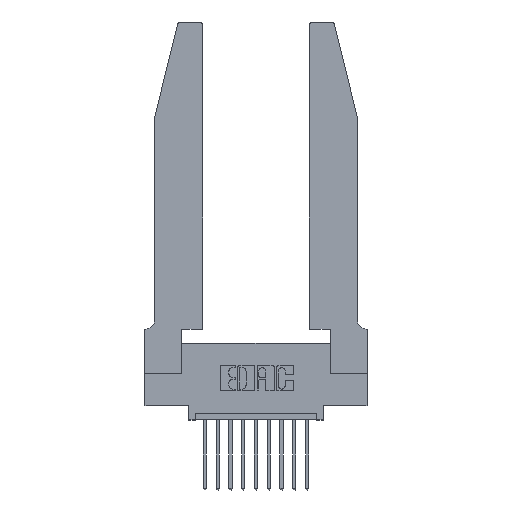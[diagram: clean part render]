
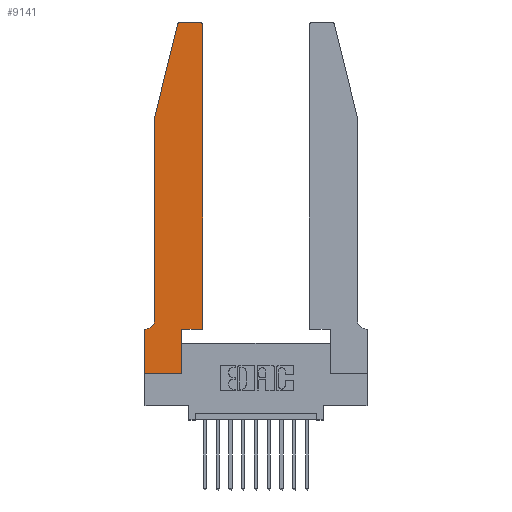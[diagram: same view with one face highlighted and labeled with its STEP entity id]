
A CAD part, top view. The second image highlights one B-rep face of the part: STEP entity #9141.
In plain terms, the highlighted planar face has unit normal (0, 0, 1).
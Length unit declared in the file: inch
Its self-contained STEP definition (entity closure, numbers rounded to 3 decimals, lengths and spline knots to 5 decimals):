
#123 = VECTOR ( 'NONE', #8610, 39.37008 ) ;
#129 = DIRECTION ( 'NONE',  ( -0.239, -0.971, 0. ) ) ;
#259 = ORIENTED_EDGE ( 'NONE', *, *, #3892, .T. ) ;
#424 = AXIS2_PLACEMENT_3D ( 'NONE', #13487, #7077, #10950 ) ;
#572 = EDGE_CURVE ( 'NONE', #2619, #15729, #4001, .T. ) ;
#602 = LINE ( 'NONE', #15996, #10327 ) ;
#708 = CARTESIAN_POINT ( 'NONE',  ( 0.0755, 0.42, 0.37 ) ) ;
#1080 = EDGE_CURVE ( 'NONE', #6767, #2516, #15290, .T. ) ;
#1112 = DIRECTION ( 'NONE',  ( 0., -1., 0. ) ) ;
#1384 = ORIENTED_EDGE ( 'NONE', *, *, #2232, .T. ) ;
#1392 = CARTESIAN_POINT ( 'NONE',  ( 0.284, 2.75, 0.37 ) ) ;
#1560 = CARTESIAN_POINT ( 'NONE',  ( 0.0055, 0.35, 0.37 ) ) ;
#1568 = VERTEX_POINT ( 'NONE', #708 ) ;
#1604 = VECTOR ( 'NONE', #12447, 39.37008 ) ;
#2035 = CARTESIAN_POINT ( 'NONE',  ( 0.0755, 2., 0.37 ) ) ;
#2090 = EDGE_CURVE ( 'NONE', #6805, #8335, #14498, .T. ) ;
#2190 = CARTESIAN_POINT ( 'NONE',  ( 0.4505, 0.35, 0.37 ) ) ;
#2211 = EDGE_LOOP ( 'NONE', ( #6377, #2398, #7430, #259, #9019, #11059, #11183, #1384, #7874, #5995, #8730, #14293 ) ) ;
#2232 = EDGE_CURVE ( 'NONE', #2516, #8833, #6122, .T. ) ;
#2398 = ORIENTED_EDGE ( 'NONE', *, *, #12355, .T. ) ;
#2414 = VECTOR ( 'NONE', #3822, 39.37008 ) ;
#2433 = LINE ( 'NONE', #3524, #16094 ) ;
#2443 = CARTESIAN_POINT ( 'NONE',  ( 0.25487, 2.72718, 0.37 ) ) ;
#2489 = CARTESIAN_POINT ( 'NONE',  ( 0.0755, 0.35, 0.37 ) ) ;
#2516 = VERTEX_POINT ( 'NONE', #11698 ) ;
#2619 = VERTEX_POINT ( 'NONE', #15563 ) ;
#2877 = DIRECTION ( 'NONE',  ( 0., 0., 1. ) ) ;
#2890 = EDGE_CURVE ( 'NONE', #13653, #11771, #15838, .T. ) ;
#3061 = CARTESIAN_POINT ( 'NONE',  ( 0.0055, 0.42, 0.37 ) ) ;
#3179 = DIRECTION ( 'NONE',  ( 0., -1., 0. ) ) ;
#3524 = CARTESIAN_POINT ( 'NONE',  ( 0.2865, 0.35, 0.37 ) ) ;
#3822 = DIRECTION ( 'NONE',  ( -1., 0., 0. ) ) ;
#3892 = EDGE_CURVE ( 'NONE', #11771, #1568, #602, .T. ) ;
#4001 = LINE ( 'NONE', #2190, #4210 ) ;
#4210 = VECTOR ( 'NONE', #12067, 39.37008 ) ;
#4375 = VECTOR ( 'NONE', #3179, 39.37008 ) ;
#4435 = DIRECTION ( 'NONE',  ( 0., 0., -1. ) ) ;
#4897 = AXIS2_PLACEMENT_3D ( 'NONE', #3061, #4435, #8191 ) ;
#5156 = VECTOR ( 'NONE', #15316, 39.37008 ) ;
#5210 = AXIS2_PLACEMENT_3D ( 'NONE', #15967, #7349, #8511 ) ;
#5339 = PLANE ( 'NONE',  #11148 ) ;
#5579 = CARTESIAN_POINT ( 'NONE',  ( 0.4205, 2.75, 0.37 ) ) ;
#5995 = ORIENTED_EDGE ( 'NONE', *, *, #572, .T. ) ;
#6122 = LINE ( 'NONE', #15006, #1604 ) ;
#6377 = ORIENTED_EDGE ( 'NONE', *, *, #6647, .T. ) ;
#6529 = LINE ( 'NONE', #6587, #5156 ) ;
#6587 = CARTESIAN_POINT ( 'NONE',  ( 0.4505, 0.35, 0.37 ) ) ;
#6647 = EDGE_CURVE ( 'NONE', #8335, #8070, #15917, .T. ) ;
#6732 = EDGE_CURVE ( 'NONE', #8833, #2619, #2433, .T. ) ;
#6767 = VERTEX_POINT ( 'NONE', #12322 ) ;
#6805 = VERTEX_POINT ( 'NONE', #12632 ) ;
#7077 = DIRECTION ( 'NONE',  ( 0., 0., 1. ) ) ;
#7330 = CARTESIAN_POINT ( 'NONE',  ( 0.2605, 2.75, 0.37 ) ) ;
#7349 = DIRECTION ( 'NONE',  ( 0., 0., 1. ) ) ;
#7430 = ORIENTED_EDGE ( 'NONE', *, *, #2890, .T. ) ;
#7783 = CARTESIAN_POINT ( 'NONE',  ( 0., 0.35, 0.37 ) ) ;
#7874 = ORIENTED_EDGE ( 'NONE', *, *, #6732, .T. ) ;
#7917 = CIRCLE ( 'NONE', #4897, 0.07 ) ;
#8070 = VERTEX_POINT ( 'NONE', #1392 ) ;
#8191 = DIRECTION ( 'NONE',  ( -1., 0., 0. ) ) ;
#8335 = VERTEX_POINT ( 'NONE', #5579 ) ;
#8511 = DIRECTION ( 'NONE',  ( 1., 0., 0. ) ) ;
#8610 = DIRECTION ( 'NONE',  ( -1., 0., 0. ) ) ;
#8642 = VERTEX_POINT ( 'NONE', #1560 ) ;
#8700 = CARTESIAN_POINT ( 'NONE',  ( 0.0755, 2., 0.37 ) ) ;
#8730 = ORIENTED_EDGE ( 'NONE', *, *, #10810, .T. ) ;
#8820 = CIRCLE ( 'NONE', #5210, 0.03 ) ;
#8833 = VERTEX_POINT ( 'NONE', #15990 ) ;
#9019 = ORIENTED_EDGE ( 'NONE', *, *, #9876, .T. ) ;
#9141 = ADVANCED_FACE ( 'NONE', ( #10471 ), #5339, .T. ) ;
#9393 = CARTESIAN_POINT ( 'NONE',  ( 0., 0., 0.37 ) ) ;
#9876 = EDGE_CURVE ( 'NONE', #1568, #8642, #7917, .T. ) ;
#9982 = VECTOR ( 'NONE', #129, 39.37008 ) ;
#10327 = VECTOR ( 'NONE', #1112, 39.37008 ) ;
#10471 = FACE_OUTER_BOUND ( 'NONE', #2211, .T. ) ;
#10810 = EDGE_CURVE ( 'NONE', #15729, #6805, #6529, .T. ) ;
#10950 = DIRECTION ( 'NONE',  ( 1., 0., 0. ) ) ;
#11059 = ORIENTED_EDGE ( 'NONE', *, *, #16037, .T. ) ;
#11148 = AXIS2_PLACEMENT_3D ( 'NONE', #7783, #2877, #12844 ) ;
#11183 = ORIENTED_EDGE ( 'NONE', *, *, #1080, .T. ) ;
#11454 = CARTESIAN_POINT ( 'NONE',  ( 0.4505, 0.35, 0.37 ) ) ;
#11698 = CARTESIAN_POINT ( 'NONE',  ( 0., 0., 0.37 ) ) ;
#11771 = VERTEX_POINT ( 'NONE', #2035 ) ;
#12067 = DIRECTION ( 'NONE',  ( 1., 0., 0. ) ) ;
#12322 = CARTESIAN_POINT ( 'NONE',  ( 0., 0.35, 0.37 ) ) ;
#12355 = EDGE_CURVE ( 'NONE', #8070, #13653, #8820, .T. ) ;
#12447 = DIRECTION ( 'NONE',  ( 1., 0., 0. ) ) ;
#12632 = CARTESIAN_POINT ( 'NONE',  ( 0.4505, 2.72, 0.37 ) ) ;
#12844 = DIRECTION ( 'NONE',  ( 1., 0., 0. ) ) ;
#13411 = DIRECTION ( 'NONE',  ( 0., 1., 0. ) ) ;
#13487 = CARTESIAN_POINT ( 'NONE',  ( 0.4205, 2.72, 0.37 ) ) ;
#13653 = VERTEX_POINT ( 'NONE', #2443 ) ;
#14079 = LINE ( 'NONE', #2489, #2414 ) ;
#14293 = ORIENTED_EDGE ( 'NONE', *, *, #2090, .T. ) ;
#14498 = CIRCLE ( 'NONE', #424, 0.03 ) ;
#15006 = CARTESIAN_POINT ( 'NONE',  ( 0., 0., 0.37 ) ) ;
#15290 = LINE ( 'NONE', #9393, #4375 ) ;
#15316 = DIRECTION ( 'NONE',  ( 0., 1., 0. ) ) ;
#15563 = CARTESIAN_POINT ( 'NONE',  ( 0.2865, 0.35, 0.37 ) ) ;
#15729 = VERTEX_POINT ( 'NONE', #11454 ) ;
#15838 = LINE ( 'NONE', #8700, #9982 ) ;
#15917 = LINE ( 'NONE', #7330, #123 ) ;
#15967 = CARTESIAN_POINT ( 'NONE',  ( 0.284, 2.72, 0.37 ) ) ;
#15990 = CARTESIAN_POINT ( 'NONE',  ( 0.2865, 0., 0.37 ) ) ;
#15996 = CARTESIAN_POINT ( 'NONE',  ( 0.0755, 2., 0.37 ) ) ;
#16037 = EDGE_CURVE ( 'NONE', #8642, #6767, #14079, .T. ) ;
#16094 = VECTOR ( 'NONE', #13411, 39.37008 ) ;
